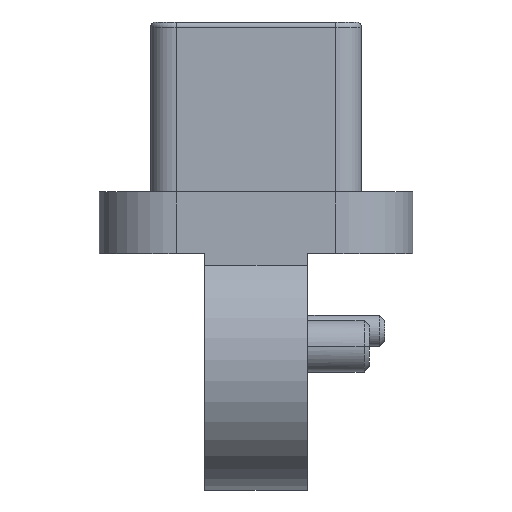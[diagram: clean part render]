
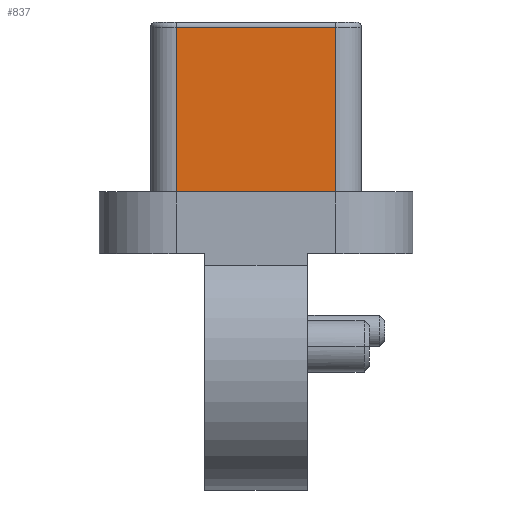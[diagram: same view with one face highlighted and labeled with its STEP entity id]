
A CAD part, left-side view. The second image highlights one B-rep face of the part: STEP entity #837.
In plain terms, the highlighted planar face has unit normal (-1, 0, 0).
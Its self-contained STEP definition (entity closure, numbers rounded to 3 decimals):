
#66 = VECTOR ( 'NONE', #5684, 1000. ) ;
#128 = EDGE_CURVE ( 'NONE', #4477, #5131, #5632, .T. ) ;
#340 = LINE ( 'NONE', #3017, #66 ) ;
#553 = VECTOR ( 'NONE', #2310, 1000. ) ;
#571 = PLANE ( 'NONE',  #4259 ) ;
#837 = ADVANCED_FACE ( 'NONE', ( #6564 ), #571, .F. ) ;
#1261 = LINE ( 'NONE', #3920, #8185 ) ;
#1376 = EDGE_CURVE ( 'NONE', #5131, #2129, #8600, .T. ) ;
#2129 = VERTEX_POINT ( 'NONE', #7429 ) ;
#2310 = DIRECTION ( 'NONE',  ( 0., 0., -1. ) ) ;
#2620 = CARTESIAN_POINT ( 'NONE',  ( -9.65, 1.55, -3.3 ) ) ;
#2819 = CARTESIAN_POINT ( 'NONE',  ( -9.65, -1.55, -0.1 ) ) ;
#2956 = CARTESIAN_POINT ( 'NONE',  ( -9.65, 1.55, -0.1 ) ) ;
#3017 = CARTESIAN_POINT ( 'NONE',  ( -9.65, -1.55, -0.1 ) ) ;
#3198 = ORIENTED_EDGE ( 'NONE', *, *, #1376, .T. ) ;
#3234 = CARTESIAN_POINT ( 'NONE',  ( -9.65, 0., -1.7 ) ) ;
#3643 = EDGE_LOOP ( 'NONE', ( #7967, #3198, #8097, #5405 ) ) ;
#3920 = CARTESIAN_POINT ( 'NONE',  ( -9.65, -1.55, -3.3 ) ) ;
#4259 = AXIS2_PLACEMENT_3D ( 'NONE', #3234, #5909, #8566 ) ;
#4477 = VERTEX_POINT ( 'NONE', #2956 ) ;
#4961 = VECTOR ( 'NONE', #5267, 1000. ) ;
#4993 = CARTESIAN_POINT ( 'NONE',  ( -9.65, 1.55, -3.3 ) ) ;
#5131 = VERTEX_POINT ( 'NONE', #4993 ) ;
#5267 = DIRECTION ( 'NONE',  ( 0., -1., 0. ) ) ;
#5405 = ORIENTED_EDGE ( 'NONE', *, *, #7567, .T. ) ;
#5632 = LINE ( 'NONE', #8293, #553 ) ;
#5684 = DIRECTION ( 'NONE',  ( 0., 1., 0. ) ) ;
#5909 = DIRECTION ( 'NONE',  ( 1., 0., 0. ) ) ;
#5933 = VERTEX_POINT ( 'NONE', #2819 ) ;
#6564 = FACE_OUTER_BOUND ( 'NONE', #3643, .T. ) ;
#6593 = DIRECTION ( 'NONE',  ( 0., 0., 1. ) ) ;
#7429 = CARTESIAN_POINT ( 'NONE',  ( -9.65, -1.55, -3.3 ) ) ;
#7567 = EDGE_CURVE ( 'NONE', #5933, #4477, #340, .T. ) ;
#7733 = EDGE_CURVE ( 'NONE', #2129, #5933, #1261, .T. ) ;
#7967 = ORIENTED_EDGE ( 'NONE', *, *, #128, .T. ) ;
#8097 = ORIENTED_EDGE ( 'NONE', *, *, #7733, .T. ) ;
#8185 = VECTOR ( 'NONE', #6593, 1000. ) ;
#8293 = CARTESIAN_POINT ( 'NONE',  ( -9.65, 1.55, -0.1 ) ) ;
#8566 = DIRECTION ( 'NONE',  ( 0., 1., 0. ) ) ;
#8600 = LINE ( 'NONE', #2620, #4961 ) ;
